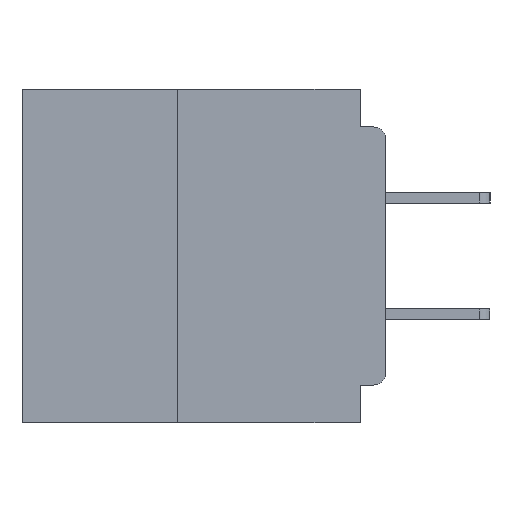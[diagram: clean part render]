
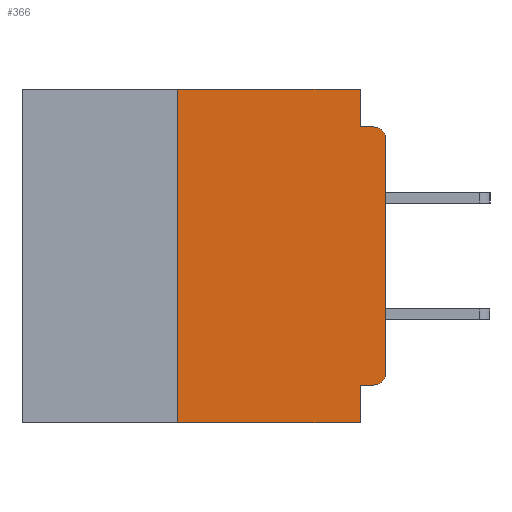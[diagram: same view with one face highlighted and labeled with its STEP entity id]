
A CAD part, left-side view. The second image highlights one B-rep face of the part: STEP entity #366.
In plain terms, the highlighted planar face has unit normal (-1, 0, 0).
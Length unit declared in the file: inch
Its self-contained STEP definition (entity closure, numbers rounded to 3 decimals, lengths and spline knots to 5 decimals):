
#366 = ADVANCED_FACE ( 'NONE', ( #34300 ), #5375, .F. ) ;
#489 = AXIS2_PLACEMENT_3D ( 'NONE', #21088, #2797, #24097 ) ;
#728 = ORIENTED_EDGE ( 'NONE', *, *, #18646, .T. ) ;
#758 = LINE ( 'NONE', #22924, #23212 ) ;
#2701 = DIRECTION ( 'NONE',  ( 0., 0., -1. ) ) ;
#2797 = DIRECTION ( 'NONE',  ( -1., 0., 0. ) ) ;
#3028 = ORIENTED_EDGE ( 'NONE', *, *, #37209, .T. ) ;
#3083 = EDGE_CURVE ( 'NONE', #9080, #19486, #20623, .T. ) ;
#4164 = DIRECTION ( 'NONE',  ( 1., 0., 0. ) ) ;
#4367 = EDGE_CURVE ( 'NONE', #27478, #24102, #33355, .T. ) ;
#4756 = LINE ( 'NONE', #28587, #28041 ) ;
#4901 = CARTESIAN_POINT ( 'NONE',  ( 0., 0.437, 0. ) ) ;
#4946 = DIRECTION ( 'NONE',  ( 0., 0., -1. ) ) ;
#4963 = VECTOR ( 'NONE', #17119, 39.37008 ) ;
#5375 = PLANE ( 'NONE',  #33563 ) ;
#6469 = VERTEX_POINT ( 'NONE', #22625 ) ;
#9080 = VERTEX_POINT ( 'NONE', #29545 ) ;
#9313 = VECTOR ( 'NONE', #18469, 39.37008 ) ;
#9986 = LINE ( 'NONE', #20979, #26076 ) ;
#10895 = DIRECTION ( 'NONE',  ( 0., 0., -1. ) ) ;
#12016 = CARTESIAN_POINT ( 'NONE',  ( 0., 0., -0.06 ) ) ;
#12313 = EDGE_CURVE ( 'NONE', #19941, #9080, #4756, .T. ) ;
#12586 = VECTOR ( 'NONE', #28423, 39.37008 ) ;
#12620 = CIRCLE ( 'NONE', #489, 0.015 ) ;
#12865 = VERTEX_POINT ( 'NONE', #25272 ) ;
#13143 = LINE ( 'NONE', #35048, #4963 ) ;
#14474 = EDGE_LOOP ( 'NONE', ( #32950, #3028, #33731, #22991, #22840, #38981, #36168, #23639, #22433, #728 ) ) ;
#14606 = LINE ( 'NONE', #25114, #37482 ) ;
#14842 = CARTESIAN_POINT ( 'NONE',  ( 0., 0.015, -0.045 ) ) ;
#14897 = EDGE_CURVE ( 'NONE', #12865, #37008, #14606, .T. ) ;
#14913 = EDGE_CURVE ( 'NONE', #19941, #6469, #22646, .T. ) ;
#16273 = DIRECTION ( 'NONE',  ( 0., -1., 0. ) ) ;
#17119 = DIRECTION ( 'NONE',  ( 0., -1., 0. ) ) ;
#18006 = DIRECTION ( 'NONE',  ( -1., 0., 0. ) ) ;
#18469 = DIRECTION ( 'NONE',  ( 0., 0., 1. ) ) ;
#18646 = EDGE_CURVE ( 'NONE', #12865, #27478, #12620, .T. ) ;
#19486 = VERTEX_POINT ( 'NONE', #36863 ) ;
#19941 = VERTEX_POINT ( 'NONE', #36474 ) ;
#20139 = CARTESIAN_POINT ( 'NONE',  ( 0., 0., 0. ) ) ;
#20623 = LINE ( 'NONE', #28970, #12586 ) ;
#20979 = CARTESIAN_POINT ( 'NONE',  ( 0., 0.031, 0. ) ) ;
#21088 = CARTESIAN_POINT ( 'NONE',  ( 0., 0.015, -0.34 ) ) ;
#21125 = EDGE_CURVE ( 'NONE', #19486, #27199, #9986, .T. ) ;
#21736 = VECTOR ( 'NONE', #16273, 39.37008 ) ;
#22433 = ORIENTED_EDGE ( 'NONE', *, *, #14897, .F. ) ;
#22625 = CARTESIAN_POINT ( 'NONE',  ( 0., 0.031, -0.4 ) ) ;
#22646 = LINE ( 'NONE', #25246, #21736 ) ;
#22840 = ORIENTED_EDGE ( 'NONE', *, *, #3083, .F. ) ;
#22924 = CARTESIAN_POINT ( 'NONE',  ( 0., 0.031, -0.4 ) ) ;
#22991 = ORIENTED_EDGE ( 'NONE', *, *, #21125, .F. ) ;
#23212 = VECTOR ( 'NONE', #10895, 39.37008 ) ;
#23639 = ORIENTED_EDGE ( 'NONE', *, *, #28366, .F. ) ;
#24097 = DIRECTION ( 'NONE',  ( 0., 0., -1. ) ) ;
#24102 = VERTEX_POINT ( 'NONE', #12016 ) ;
#25114 = CARTESIAN_POINT ( 'NONE',  ( 0., 0., -0.355 ) ) ;
#25246 = CARTESIAN_POINT ( 'NONE',  ( 0., 0.437, -0.4 ) ) ;
#25272 = CARTESIAN_POINT ( 'NONE',  ( 0., 0.015, -0.355 ) ) ;
#25571 = DIRECTION ( 'NONE',  ( 0., 0., 1. ) ) ;
#26076 = VECTOR ( 'NONE', #2701, 39.37008 ) ;
#27199 = VERTEX_POINT ( 'NONE', #29331 ) ;
#27478 = VERTEX_POINT ( 'NONE', #27734 ) ;
#27734 = CARTESIAN_POINT ( 'NONE',  ( 0., 0., -0.34 ) ) ;
#28041 = VECTOR ( 'NONE', #25571, 39.37008 ) ;
#28135 = CIRCLE ( 'NONE', #34405, 0.015 ) ;
#28259 = DIRECTION ( 'NONE',  ( 0., 1., 0. ) ) ;
#28366 = EDGE_CURVE ( 'NONE', #37008, #6469, #758, .T. ) ;
#28423 = DIRECTION ( 'NONE',  ( 0., -1., 0. ) ) ;
#28587 = CARTESIAN_POINT ( 'NONE',  ( 0., 0.25, -0.4 ) ) ;
#28970 = CARTESIAN_POINT ( 'NONE',  ( 0., 0.437, 0. ) ) ;
#29331 = CARTESIAN_POINT ( 'NONE',  ( 0., 0.031, -0.045 ) ) ;
#29545 = CARTESIAN_POINT ( 'NONE',  ( 0., 0.25, 0. ) ) ;
#30230 = EDGE_CURVE ( 'NONE', #27199, #37710, #13143, .T. ) ;
#32044 = CARTESIAN_POINT ( 'NONE',  ( 0., 0.031, -0.355 ) ) ;
#32950 = ORIENTED_EDGE ( 'NONE', *, *, #4367, .T. ) ;
#33355 = LINE ( 'NONE', #20139, #9313 ) ;
#33563 = AXIS2_PLACEMENT_3D ( 'NONE', #4901, #4164, #4946 ) ;
#33731 = ORIENTED_EDGE ( 'NONE', *, *, #30230, .F. ) ;
#34300 = FACE_OUTER_BOUND ( 'NONE', #14474, .T. ) ;
#34405 = AXIS2_PLACEMENT_3D ( 'NONE', #35880, #18006, #38806 ) ;
#35048 = CARTESIAN_POINT ( 'NONE',  ( 0., 0., -0.045 ) ) ;
#35880 = CARTESIAN_POINT ( 'NONE',  ( 0., 0.015, -0.06 ) ) ;
#36168 = ORIENTED_EDGE ( 'NONE', *, *, #14913, .T. ) ;
#36474 = CARTESIAN_POINT ( 'NONE',  ( 0., 0.25, -0.4 ) ) ;
#36863 = CARTESIAN_POINT ( 'NONE',  ( 0., 0.031, 0. ) ) ;
#37008 = VERTEX_POINT ( 'NONE', #32044 ) ;
#37209 = EDGE_CURVE ( 'NONE', #24102, #37710, #28135, .T. ) ;
#37482 = VECTOR ( 'NONE', #28259, 39.37008 ) ;
#37710 = VERTEX_POINT ( 'NONE', #14842 ) ;
#38806 = DIRECTION ( 'NONE',  ( 0., 0., -1. ) ) ;
#38981 = ORIENTED_EDGE ( 'NONE', *, *, #12313, .F. ) ;
